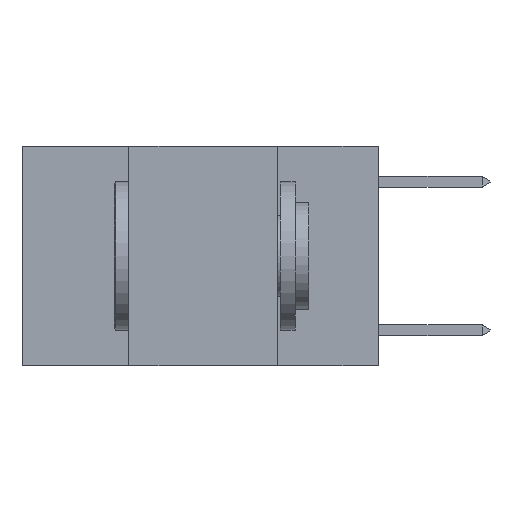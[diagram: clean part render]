
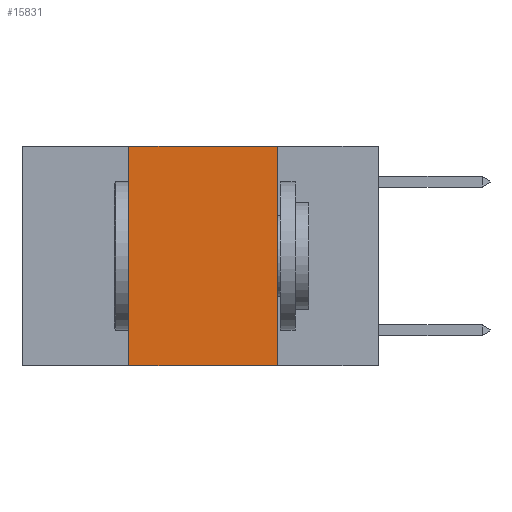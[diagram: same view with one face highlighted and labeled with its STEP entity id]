
A CAD part, left-side view. The second image highlights one B-rep face of the part: STEP entity #15831.
In plain terms, the highlighted planar face has unit normal (-1, 0, 0).
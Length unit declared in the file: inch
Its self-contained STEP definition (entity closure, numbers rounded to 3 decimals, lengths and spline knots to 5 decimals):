
#1047 = LINE ( 'NONE', #8864, #13209 ) ;
#1224 = CARTESIAN_POINT ( 'NONE',  ( 0., 0.6, 0. ) ) ;
#1245 = DIRECTION ( 'NONE',  ( 0., 0., 1. ) ) ;
#1470 = EDGE_CURVE ( 'NONE', #10078, #6433, #1047, .T. ) ;
#1789 = LINE ( 'NONE', #23194, #24365 ) ;
#2332 = ORIENTED_EDGE ( 'NONE', *, *, #1470, .T. ) ;
#2885 = PLANE ( 'NONE',  #16547 ) ;
#3398 = EDGE_CURVE ( 'NONE', #18643, #3789, #14507, .T. ) ;
#3533 = CARTESIAN_POINT ( 'NONE',  ( 0., 0.17, 0. ) ) ;
#3789 = VERTEX_POINT ( 'NONE', #3533 ) ;
#4088 = CARTESIAN_POINT ( 'NONE',  ( 0., 0.6, 0. ) ) ;
#4471 = DIRECTION ( 'NONE',  ( 0., -1., 0. ) ) ;
#6433 = VERTEX_POINT ( 'NONE', #16354 ) ;
#6791 = CARTESIAN_POINT ( 'NONE',  ( 0., 0.42, 0. ) ) ;
#6908 = DIRECTION ( 'NONE',  ( 0., -1., 0. ) ) ;
#7676 = EDGE_CURVE ( 'NONE', #3789, #6433, #1789, .T. ) ;
#8286 = VECTOR ( 'NONE', #1245, 39.37008 ) ;
#8864 = CARTESIAN_POINT ( 'NONE',  ( 0., 0.6, -0.37 ) ) ;
#10078 = VERTEX_POINT ( 'NONE', #13051 ) ;
#10988 = LINE ( 'NONE', #16609, #8286 ) ;
#11934 = ORIENTED_EDGE ( 'NONE', *, *, #7676, .F. ) ;
#13051 = CARTESIAN_POINT ( 'NONE',  ( 0., 0.42, -0.37 ) ) ;
#13209 = VECTOR ( 'NONE', #6908, 39.37008 ) ;
#13588 = DIRECTION ( 'NONE',  ( 0., 0., -1. ) ) ;
#14507 = LINE ( 'NONE', #4088, #24426 ) ;
#15066 = DIRECTION ( 'NONE',  ( 1., 0., 0. ) ) ;
#15182 = FACE_OUTER_BOUND ( 'NONE', #18579, .T. ) ;
#15831 = ADVANCED_FACE ( 'NONE', ( #15182 ), #2885, .F. ) ;
#16354 = CARTESIAN_POINT ( 'NONE',  ( 0., 0.17, -0.37 ) ) ;
#16547 = AXIS2_PLACEMENT_3D ( 'NONE', #1224, #15066, #20749 ) ;
#16609 = CARTESIAN_POINT ( 'NONE',  ( 0., 0.42, 0. ) ) ;
#18495 = EDGE_CURVE ( 'NONE', #10078, #18643, #10988, .T. ) ;
#18579 = EDGE_LOOP ( 'NONE', ( #11934, #21063, #20905, #2332 ) ) ;
#18643 = VERTEX_POINT ( 'NONE', #6791 ) ;
#20749 = DIRECTION ( 'NONE',  ( 0., 0., -1. ) ) ;
#20905 = ORIENTED_EDGE ( 'NONE', *, *, #18495, .F. ) ;
#21063 = ORIENTED_EDGE ( 'NONE', *, *, #3398, .F. ) ;
#23194 = CARTESIAN_POINT ( 'NONE',  ( 0., 0.17, 0. ) ) ;
#24365 = VECTOR ( 'NONE', #13588, 39.37008 ) ;
#24426 = VECTOR ( 'NONE', #4471, 39.37008 ) ;
